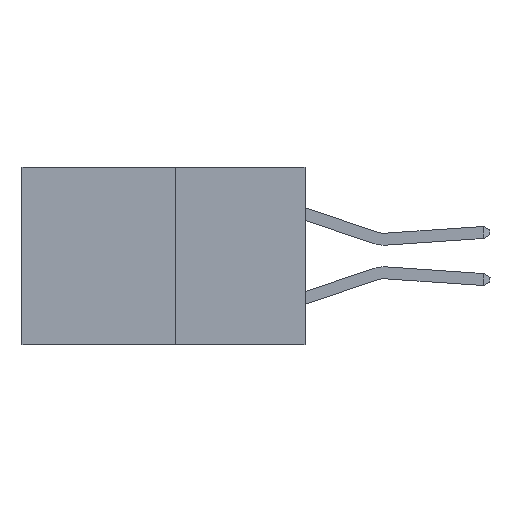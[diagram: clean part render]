
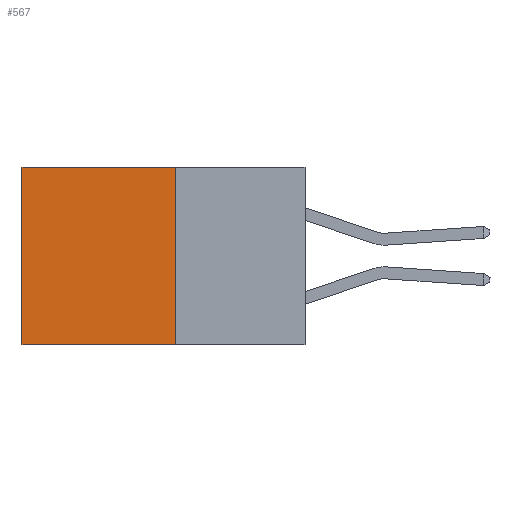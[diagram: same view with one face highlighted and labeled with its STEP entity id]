
A CAD part, left-side view. The second image highlights one B-rep face of the part: STEP entity #567.
In plain terms, the highlighted planar face has unit normal (-1, 0, 0).
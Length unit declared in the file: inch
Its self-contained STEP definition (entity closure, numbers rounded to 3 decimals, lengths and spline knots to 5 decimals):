
#481 = EDGE_CURVE ( 'NONE', #5757, #6493, #1240, .T. ) ;
#567 = ADVANCED_FACE ( 'NONE', ( #1936 ), #9401, .F. ) ;
#748 = CARTESIAN_POINT ( 'NONE',  ( 0.277, 0.27, -0.37 ) ) ;
#1232 = DIRECTION ( 'NONE',  ( 0., 0., -1. ) ) ;
#1240 = LINE ( 'NONE', #6498, #9731 ) ;
#1290 = CARTESIAN_POINT ( 'NONE',  ( 0.277, 0.59, 0. ) ) ;
#1751 = VECTOR ( 'NONE', #1232, 39.37008 ) ;
#1936 = FACE_OUTER_BOUND ( 'NONE', #3063, .T. ) ;
#2169 = VECTOR ( 'NONE', #7500, 39.37008 ) ;
#2396 = EDGE_CURVE ( 'NONE', #7504, #5757, #9178, .T. ) ;
#2720 = EDGE_CURVE ( 'NONE', #6693, #6493, #8228, .T. ) ;
#2878 = DIRECTION ( 'NONE',  ( 0., 0., -1. ) ) ;
#3063 = EDGE_LOOP ( 'NONE', ( #5771, #5817, #5830, #5900 ) ) ;
#3862 = EDGE_CURVE ( 'NONE', #7504, #6693, #8505, .T. ) ;
#5523 = DIRECTION ( 'NONE',  ( 0., 1., 0. ) ) ;
#5547 = CARTESIAN_POINT ( 'NONE',  ( 0.277, 0.27, -0.37 ) ) ;
#5757 = VERTEX_POINT ( 'NONE', #1290 ) ;
#5771 = ORIENTED_EDGE ( 'NONE', *, *, #481, .T. ) ;
#5785 = AXIS2_PLACEMENT_3D ( 'NONE', #9933, #9634, #7719 ) ;
#5817 = ORIENTED_EDGE ( 'NONE', *, *, #2720, .F. ) ;
#5830 = ORIENTED_EDGE ( 'NONE', *, *, #3862, .F. ) ;
#5900 = ORIENTED_EDGE ( 'NONE', *, *, #2396, .T. ) ;
#6208 = VECTOR ( 'NONE', #5523, 39.37008 ) ;
#6228 = CARTESIAN_POINT ( 'NONE',  ( 0.277, 0.27, -0.37 ) ) ;
#6381 = CARTESIAN_POINT ( 'NONE',  ( 0.277, 0.27, 0. ) ) ;
#6493 = VERTEX_POINT ( 'NONE', #7694 ) ;
#6498 = CARTESIAN_POINT ( 'NONE',  ( 0.277, 0.59, -0.37 ) ) ;
#6693 = VERTEX_POINT ( 'NONE', #6228 ) ;
#7500 = DIRECTION ( 'NONE',  ( 0., 1., 0. ) ) ;
#7504 = VERTEX_POINT ( 'NONE', #10856 ) ;
#7694 = CARTESIAN_POINT ( 'NONE',  ( 0.277, 0.59, -0.37 ) ) ;
#7719 = DIRECTION ( 'NONE',  ( 0., 0., -1. ) ) ;
#8228 = LINE ( 'NONE', #5547, #6208 ) ;
#8505 = LINE ( 'NONE', #748, #1751 ) ;
#9178 = LINE ( 'NONE', #6381, #2169 ) ;
#9401 = PLANE ( 'NONE',  #5785 ) ;
#9634 = DIRECTION ( 'NONE',  ( 1., 0., 0. ) ) ;
#9731 = VECTOR ( 'NONE', #2878, 39.37008 ) ;
#9933 = CARTESIAN_POINT ( 'NONE',  ( 0.277, 0.27, -0.37 ) ) ;
#10856 = CARTESIAN_POINT ( 'NONE',  ( 0.277, 0.27, 0. ) ) ;
